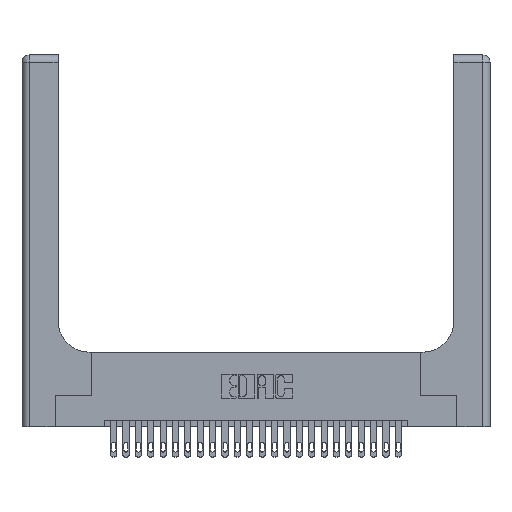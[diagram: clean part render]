
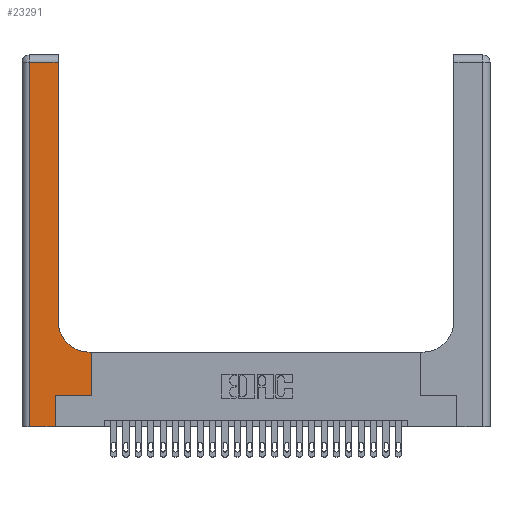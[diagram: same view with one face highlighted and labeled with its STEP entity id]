
A CAD part, top view. The second image highlights one B-rep face of the part: STEP entity #23291.
In plain terms, the highlighted planar face has unit normal (0, 0, 1).
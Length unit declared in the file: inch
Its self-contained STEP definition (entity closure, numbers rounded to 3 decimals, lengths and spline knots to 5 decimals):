
#419 = ORIENTED_EDGE ( 'NONE', *, *, #15966, .T. ) ;
#669 = CARTESIAN_POINT ( 'NONE',  ( 0., 3., 0.37 ) ) ;
#1367 = ORIENTED_EDGE ( 'NONE', *, *, #20965, .T. ) ;
#1731 = DIRECTION ( 'NONE',  ( 1., 0., 0. ) ) ;
#2069 = VECTOR ( 'NONE', #19221, 39.37008 ) ;
#2149 = LINE ( 'NONE', #18860, #9548 ) ;
#2239 = VERTEX_POINT ( 'NONE', #12732 ) ;
#2273 = EDGE_CURVE ( 'NONE', #3898, #13200, #8806, .T. ) ;
#2468 = DIRECTION ( 'NONE',  ( 1., 0., 0. ) ) ;
#2679 = EDGE_CURVE ( 'NONE', #13200, #4844, #3355, .T. ) ;
#2685 = EDGE_CURVE ( 'NONE', #11926, #11313, #10405, .T. ) ;
#2954 = CARTESIAN_POINT ( 'NONE',  ( 0.2915, 0.85, 0.37 ) ) ;
#3238 = AXIS2_PLACEMENT_3D ( 'NONE', #669, #18730, #16638 ) ;
#3270 = VECTOR ( 'NONE', #1731, 39.37008 ) ;
#3300 = CARTESIAN_POINT ( 'NONE',  ( 0.06, 2.94, 0.37 ) ) ;
#3355 = LINE ( 'NONE', #15931, #11378 ) ;
#3898 = VERTEX_POINT ( 'NONE', #11121 ) ;
#4340 = ORIENTED_EDGE ( 'NONE', *, *, #7124, .T. ) ;
#4844 = VERTEX_POINT ( 'NONE', #5389 ) ;
#5389 = CARTESIAN_POINT ( 'NONE',  ( 0.06, 0., 0.37 ) ) ;
#5472 = FACE_OUTER_BOUND ( 'NONE', #16145, .T. ) ;
#6131 = CARTESIAN_POINT ( 'NONE',  ( 0.2915, 0.6, 0.37 ) ) ;
#6784 = CARTESIAN_POINT ( 'NONE',  ( 0.269, 0., 0.37 ) ) ;
#7124 = EDGE_CURVE ( 'NONE', #26067, #2239, #24238, .T. ) ;
#8806 = LINE ( 'NONE', #21174, #2069 ) ;
#9026 = CARTESIAN_POINT ( 'NONE',  ( 0.269, 0., 0.37 ) ) ;
#9211 = EDGE_CURVE ( 'NONE', #2239, #13238, #2149, .T. ) ;
#9545 = CARTESIAN_POINT ( 'NONE',  ( 0.5585, 0.6, 0.37 ) ) ;
#9548 = VECTOR ( 'NONE', #22656, 39.37008 ) ;
#10194 = VECTOR ( 'NONE', #10239, 39.37008 ) ;
#10239 = DIRECTION ( 'NONE',  ( -1., 0., 0. ) ) ;
#10241 = VECTOR ( 'NONE', #2468, 39.37008 ) ;
#10405 = CIRCLE ( 'NONE', #24156, 0.25 ) ;
#10605 = CARTESIAN_POINT ( 'NONE',  ( 0.269, 0.25, 0.37 ) ) ;
#11121 = CARTESIAN_POINT ( 'NONE',  ( 0.2915, 2.94, 0.37 ) ) ;
#11313 = VERTEX_POINT ( 'NONE', #2954 ) ;
#11378 = VECTOR ( 'NONE', #12312, 39.37008 ) ;
#11926 = VERTEX_POINT ( 'NONE', #20591 ) ;
#12000 = DIRECTION ( 'NONE',  ( 1., 0., 0. ) ) ;
#12312 = DIRECTION ( 'NONE',  ( 0., -1., 0. ) ) ;
#12364 = EDGE_CURVE ( 'NONE', #11313, #3898, #23341, .T. ) ;
#12571 = ORIENTED_EDGE ( 'NONE', *, *, #9211, .T. ) ;
#12732 = CARTESIAN_POINT ( 'NONE',  ( 0.5585, 0.25, 0.37 ) ) ;
#13200 = VERTEX_POINT ( 'NONE', #3300 ) ;
#13238 = VERTEX_POINT ( 'NONE', #9545 ) ;
#13595 = ORIENTED_EDGE ( 'NONE', *, *, #2685, .T. ) ;
#14075 = CARTESIAN_POINT ( 'NONE',  ( 0.269, 0.25, 0.37 ) ) ;
#15183 = EDGE_CURVE ( 'NONE', #4844, #17632, #20654, .T. ) ;
#15359 = DIRECTION ( 'NONE',  ( 0., 1., 0. ) ) ;
#15931 = CARTESIAN_POINT ( 'NONE',  ( 0.06, 3., 0.37 ) ) ;
#15966 = EDGE_CURVE ( 'NONE', #13238, #11926, #23797, .T. ) ;
#16145 = EDGE_LOOP ( 'NONE', ( #18431, #22403, #17777, #24138, #1367, #4340, #12571, #419, #13595 ) ) ;
#16638 = DIRECTION ( 'NONE',  ( -1., 0., 0. ) ) ;
#16709 = VECTOR ( 'NONE', #15359, 39.37008 ) ;
#17632 = VERTEX_POINT ( 'NONE', #6784 ) ;
#17777 = ORIENTED_EDGE ( 'NONE', *, *, #2679, .T. ) ;
#17946 = VECTOR ( 'NONE', #24777, 39.37008 ) ;
#18431 = ORIENTED_EDGE ( 'NONE', *, *, #12364, .T. ) ;
#18564 = CARTESIAN_POINT ( 'NONE',  ( 0., 0., 0.37 ) ) ;
#18664 = CARTESIAN_POINT ( 'NONE',  ( 0.5415, 0.85, 0.37 ) ) ;
#18730 = DIRECTION ( 'NONE',  ( 0., 0., -1. ) ) ;
#18814 = CARTESIAN_POINT ( 'NONE',  ( 0.2915, 3., 0.37 ) ) ;
#18860 = CARTESIAN_POINT ( 'NONE',  ( 0.5585, 0.25, 0.37 ) ) ;
#19221 = DIRECTION ( 'NONE',  ( -1., 0., 0. ) ) ;
#20591 = CARTESIAN_POINT ( 'NONE',  ( 0.5415, 0.6, 0.37 ) ) ;
#20654 = LINE ( 'NONE', #18564, #10241 ) ;
#20753 = PLANE ( 'NONE',  #3238 ) ;
#20965 = EDGE_CURVE ( 'NONE', #17632, #26067, #21771, .T. ) ;
#21174 = CARTESIAN_POINT ( 'NONE',  ( 0., 2.94, 0.37 ) ) ;
#21771 = LINE ( 'NONE', #9026, #16709 ) ;
#22403 = ORIENTED_EDGE ( 'NONE', *, *, #2273, .T. ) ;
#22656 = DIRECTION ( 'NONE',  ( 0., 1., 0. ) ) ;
#23291 = ADVANCED_FACE ( 'NONE', ( #5472 ), #20753, .F. ) ;
#23341 = LINE ( 'NONE', #18814, #17946 ) ;
#23797 = LINE ( 'NONE', #6131, #10194 ) ;
#24138 = ORIENTED_EDGE ( 'NONE', *, *, #15183, .T. ) ;
#24156 = AXIS2_PLACEMENT_3D ( 'NONE', #18664, #26391, #12000 ) ;
#24238 = LINE ( 'NONE', #14075, #3270 ) ;
#24777 = DIRECTION ( 'NONE',  ( 0., 1., 0. ) ) ;
#26067 = VERTEX_POINT ( 'NONE', #10605 ) ;
#26391 = DIRECTION ( 'NONE',  ( 0., 0., -1. ) ) ;
